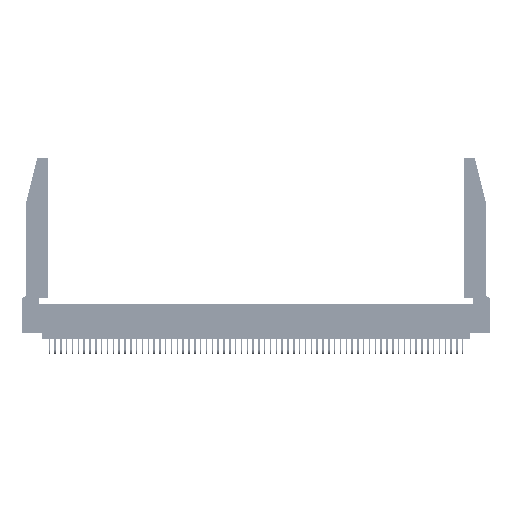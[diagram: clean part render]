
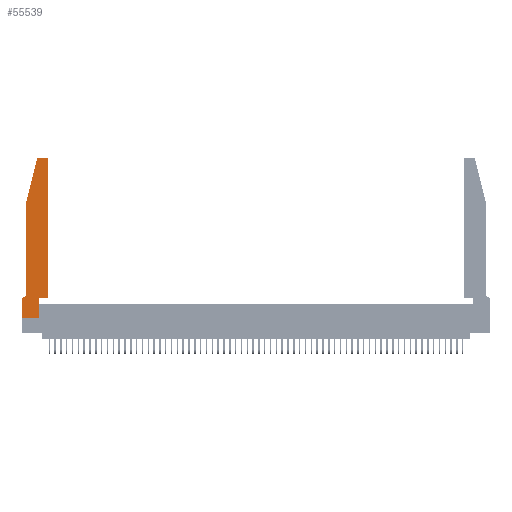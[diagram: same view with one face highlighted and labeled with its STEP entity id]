
A CAD part, top view. The second image highlights one B-rep face of the part: STEP entity #55539.
In plain terms, the highlighted planar face has unit normal (0, 0, 1).
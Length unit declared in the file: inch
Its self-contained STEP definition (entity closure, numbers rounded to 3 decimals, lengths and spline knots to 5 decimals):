
#11 = DIRECTION ( 'NONE',  ( 1., 0., 0. ) ) ;
#614 = DIRECTION ( 'NONE',  ( 1., 0., 0. ) ) ;
#1084 = AXIS2_PLACEMENT_3D ( 'NONE', #2393, #38968, #11734 ) ;
#1550 = CARTESIAN_POINT ( 'NONE',  ( 0.0755, 2., 0.37 ) ) ;
#1757 = VERTEX_POINT ( 'NONE', #13669 ) ;
#1981 = CARTESIAN_POINT ( 'NONE',  ( 0.0755, 2., 0.37 ) ) ;
#2016 = ORIENTED_EDGE ( 'NONE', *, *, #51465, .T. ) ;
#2126 = ORIENTED_EDGE ( 'NONE', *, *, #48166, .T. ) ;
#2393 = CARTESIAN_POINT ( 'NONE',  ( 0.284, 2.72, 0.37 ) ) ;
#2450 = DIRECTION ( 'NONE',  ( 0., 1., 0. ) ) ;
#2839 = CARTESIAN_POINT ( 'NONE',  ( 0., 0.35, 0.37 ) ) ;
#3201 = CARTESIAN_POINT ( 'NONE',  ( 0., 0., 0.37 ) ) ;
#3528 = DIRECTION ( 'NONE',  ( 0., 0., -1. ) ) ;
#4422 = CARTESIAN_POINT ( 'NONE',  ( 0.25487, 2.72718, 0.37 ) ) ;
#5105 = EDGE_CURVE ( 'NONE', #40094, #37410, #32580, .T. ) ;
#5984 = CARTESIAN_POINT ( 'NONE',  ( 0.2865, 0., 0.37 ) ) ;
#6737 = CARTESIAN_POINT ( 'NONE',  ( 0.4505, 0.35, 0.37 ) ) ;
#6979 = VERTEX_POINT ( 'NONE', #39905 ) ;
#6989 = VECTOR ( 'NONE', #48584, 39.37008 ) ;
#9574 = EDGE_LOOP ( 'NONE', ( #18914, #41986, #11072, #40169, #30213, #47979, #15289, #32866, #2016, #42766, #15703, #2126 ) ) ;
#10247 = LINE ( 'NONE', #56000, #46545 ) ;
#11072 = ORIENTED_EDGE ( 'NONE', *, *, #47243, .T. ) ;
#11086 = VERTEX_POINT ( 'NONE', #23425 ) ;
#11734 = DIRECTION ( 'NONE',  ( 1., 0., 0. ) ) ;
#13104 = DIRECTION ( 'NONE',  ( 1., 0., 0. ) ) ;
#13669 = CARTESIAN_POINT ( 'NONE',  ( 0.2865, 0.35, 0.37 ) ) ;
#14322 = CARTESIAN_POINT ( 'NONE',  ( 0., 0., 0.37 ) ) ;
#14410 = EDGE_CURVE ( 'NONE', #14747, #15867, #56248, .T. ) ;
#14747 = VERTEX_POINT ( 'NONE', #38173 ) ;
#14916 = VECTOR ( 'NONE', #40401, 39.37008 ) ;
#15171 = DIRECTION ( 'NONE',  ( -0.239, -0.971, 0. ) ) ;
#15289 = ORIENTED_EDGE ( 'NONE', *, *, #55157, .T. ) ;
#15703 = ORIENTED_EDGE ( 'NONE', *, *, #5105, .T. ) ;
#15794 = CARTESIAN_POINT ( 'NONE',  ( 0.0755, 0.42, 0.37 ) ) ;
#15867 = VERTEX_POINT ( 'NONE', #26915 ) ;
#17300 = VECTOR ( 'NONE', #2450, 39.37008 ) ;
#18914 = ORIENTED_EDGE ( 'NONE', *, *, #14410, .T. ) ;
#19698 = VERTEX_POINT ( 'NONE', #4422 ) ;
#19741 = EDGE_CURVE ( 'NONE', #6979, #25062, #25012, .T. ) ;
#20191 = CARTESIAN_POINT ( 'NONE',  ( 0.2865, 0.35, 0.37 ) ) ;
#20968 = DIRECTION ( 'NONE',  ( 1., 0., 0. ) ) ;
#21146 = FACE_OUTER_BOUND ( 'NONE', #9574, .T. ) ;
#21448 = CARTESIAN_POINT ( 'NONE',  ( 0.0055, 0.42, 0.37 ) ) ;
#22687 = PLANE ( 'NONE',  #41754 ) ;
#22726 = VERTEX_POINT ( 'NONE', #2839 ) ;
#23425 = CARTESIAN_POINT ( 'NONE',  ( 0.0055, 0.35, 0.37 ) ) ;
#24417 = CIRCLE ( 'NONE', #35980, 0.07 ) ;
#25012 = LINE ( 'NONE', #14322, #38544 ) ;
#25062 = VERTEX_POINT ( 'NONE', #5984 ) ;
#26421 = DIRECTION ( 'NONE',  ( 0., 0., 1. ) ) ;
#26915 = CARTESIAN_POINT ( 'NONE',  ( 0.284, 2.75, 0.37 ) ) ;
#27058 = CARTESIAN_POINT ( 'NONE',  ( 0.4505, 0.35, 0.37 ) ) ;
#27229 = DIRECTION ( 'NONE',  ( 0., 0., 1. ) ) ;
#29291 = LINE ( 'NONE', #1550, #36420 ) ;
#30213 = ORIENTED_EDGE ( 'NONE', *, *, #31140, .T. ) ;
#31140 = EDGE_CURVE ( 'NONE', #39872, #11086, #24417, .T. ) ;
#31146 = LINE ( 'NONE', #3201, #6989 ) ;
#32075 = LINE ( 'NONE', #42756, #36351 ) ;
#32580 = LINE ( 'NONE', #6737, #46126 ) ;
#32866 = ORIENTED_EDGE ( 'NONE', *, *, #19741, .T. ) ;
#32882 = CIRCLE ( 'NONE', #52602, 0.03 ) ;
#35071 = LINE ( 'NONE', #20191, #17300 ) ;
#35980 = AXIS2_PLACEMENT_3D ( 'NONE', #21448, #3528, #57706 ) ;
#36351 = VECTOR ( 'NONE', #51978, 39.37008 ) ;
#36420 = VECTOR ( 'NONE', #39283, 39.37008 ) ;
#37410 = VERTEX_POINT ( 'NONE', #37969 ) ;
#37969 = CARTESIAN_POINT ( 'NONE',  ( 0.4505, 2.72, 0.37 ) ) ;
#38173 = CARTESIAN_POINT ( 'NONE',  ( 0.4205, 2.75, 0.37 ) ) ;
#38544 = VECTOR ( 'NONE', #614, 39.37008 ) ;
#38968 = DIRECTION ( 'NONE',  ( 0., 0., 1. ) ) ;
#39283 = DIRECTION ( 'NONE',  ( 0., -1., 0. ) ) ;
#39872 = VERTEX_POINT ( 'NONE', #15794 ) ;
#39905 = CARTESIAN_POINT ( 'NONE',  ( 0., 0., 0.37 ) ) ;
#39947 = CARTESIAN_POINT ( 'NONE',  ( 0.4205, 2.72, 0.37 ) ) ;
#40094 = VERTEX_POINT ( 'NONE', #27058 ) ;
#40169 = ORIENTED_EDGE ( 'NONE', *, *, #48617, .T. ) ;
#40401 = DIRECTION ( 'NONE',  ( -1., 0., 0. ) ) ;
#41754 = AXIS2_PLACEMENT_3D ( 'NONE', #46137, #27229, #11 ) ;
#41986 = ORIENTED_EDGE ( 'NONE', *, *, #58804, .T. ) ;
#42756 = CARTESIAN_POINT ( 'NONE',  ( 0.0755, 0.35, 0.37 ) ) ;
#42766 = ORIENTED_EDGE ( 'NONE', *, *, #51587, .T. ) ;
#43506 = DIRECTION ( 'NONE',  ( 0., 1., 0. ) ) ;
#46055 = VERTEX_POINT ( 'NONE', #1981 ) ;
#46126 = VECTOR ( 'NONE', #43506, 39.37008 ) ;
#46137 = CARTESIAN_POINT ( 'NONE',  ( 0., 0.35, 0.37 ) ) ;
#46545 = VECTOR ( 'NONE', #15171, 39.37008 ) ;
#47003 = CIRCLE ( 'NONE', #1084, 0.03 ) ;
#47243 = EDGE_CURVE ( 'NONE', #19698, #46055, #10247, .T. ) ;
#47834 = CARTESIAN_POINT ( 'NONE',  ( 0.4505, 0.35, 0.37 ) ) ;
#47979 = ORIENTED_EDGE ( 'NONE', *, *, #58626, .T. ) ;
#48166 = EDGE_CURVE ( 'NONE', #37410, #14747, #32882, .T. ) ;
#48584 = DIRECTION ( 'NONE',  ( 0., -1., 0. ) ) ;
#48617 = EDGE_CURVE ( 'NONE', #46055, #39872, #29291, .T. ) ;
#48637 = LINE ( 'NONE', #47834, #55058 ) ;
#51465 = EDGE_CURVE ( 'NONE', #25062, #1757, #35071, .T. ) ;
#51587 = EDGE_CURVE ( 'NONE', #1757, #40094, #48637, .T. ) ;
#51978 = DIRECTION ( 'NONE',  ( -1., 0., 0. ) ) ;
#52602 = AXIS2_PLACEMENT_3D ( 'NONE', #39947, #26421, #13104 ) ;
#53999 = CARTESIAN_POINT ( 'NONE',  ( 0.2605, 2.75, 0.37 ) ) ;
#55058 = VECTOR ( 'NONE', #20968, 39.37008 ) ;
#55157 = EDGE_CURVE ( 'NONE', #22726, #6979, #31146, .T. ) ;
#55539 = ADVANCED_FACE ( 'NONE', ( #21146 ), #22687, .T. ) ;
#56000 = CARTESIAN_POINT ( 'NONE',  ( 0.0755, 2., 0.37 ) ) ;
#56248 = LINE ( 'NONE', #53999, #14916 ) ;
#57706 = DIRECTION ( 'NONE',  ( -1., 0., 0. ) ) ;
#58626 = EDGE_CURVE ( 'NONE', #11086, #22726, #32075, .T. ) ;
#58804 = EDGE_CURVE ( 'NONE', #15867, #19698, #47003, .T. ) ;
